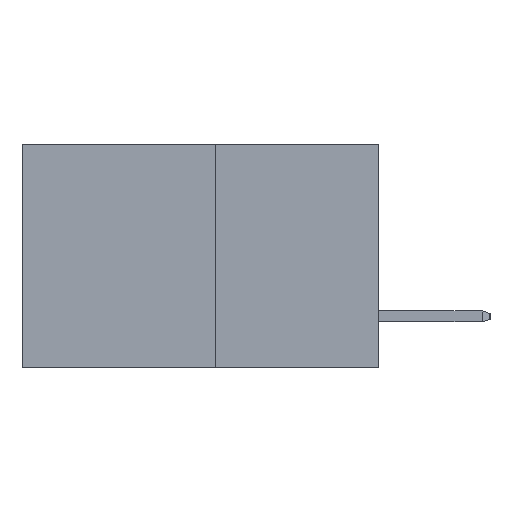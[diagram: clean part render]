
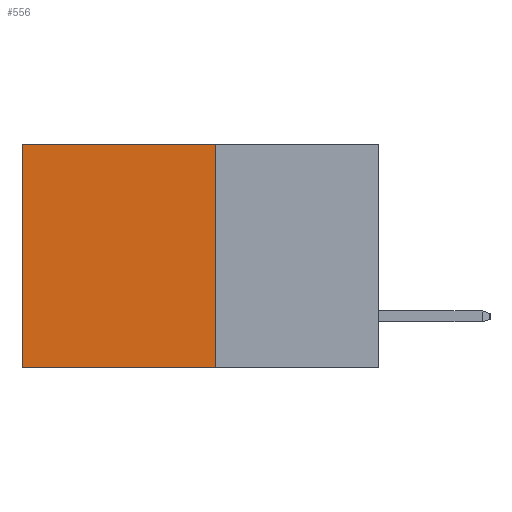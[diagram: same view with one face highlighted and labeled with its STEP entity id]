
A CAD part, left-side view. The second image highlights one B-rep face of the part: STEP entity #556.
In plain terms, the highlighted planar face has unit normal (-1, 0, 0).
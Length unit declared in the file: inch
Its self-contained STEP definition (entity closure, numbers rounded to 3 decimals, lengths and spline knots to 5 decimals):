
#320 = VERTEX_POINT ( 'NONE', #10643 ) ;
#556 = ADVANCED_FACE ( 'NONE', ( #1606 ), #7181, .F. ) ;
#638 = DIRECTION ( 'NONE',  ( 0., 0., -1. ) ) ;
#1606 = FACE_OUTER_BOUND ( 'NONE', #9519, .T. ) ;
#1773 = EDGE_CURVE ( 'NONE', #8562, #7394, #2162, .T. ) ;
#1895 = DIRECTION ( 'NONE',  ( 1., 0., 0. ) ) ;
#2162 = LINE ( 'NONE', #6145, #2445 ) ;
#2347 = LINE ( 'NONE', #3818, #9650 ) ;
#2445 = VECTOR ( 'NONE', #6106, 39.37008 ) ;
#2896 = ORIENTED_EDGE ( 'NONE', *, *, #3645, .T. ) ;
#3191 = ORIENTED_EDGE ( 'NONE', *, *, #10747, .T. ) ;
#3645 = EDGE_CURVE ( 'NONE', #320, #7394, #4684, .T. ) ;
#3818 = CARTESIAN_POINT ( 'NONE',  ( 0.277, 0.27, 0. ) ) ;
#4272 = CARTESIAN_POINT ( 'NONE',  ( 0.277, 0.27, -0.37 ) ) ;
#4500 = VERTEX_POINT ( 'NONE', #7569 ) ;
#4599 = LINE ( 'NONE', #6150, #9473 ) ;
#4684 = LINE ( 'NONE', #7059, #11668 ) ;
#5683 = CARTESIAN_POINT ( 'NONE',  ( 0.277, 0.59, -0.37 ) ) ;
#6106 = DIRECTION ( 'NONE',  ( 0., 1., 0. ) ) ;
#6145 = CARTESIAN_POINT ( 'NONE',  ( 0.277, 0.27, -0.37 ) ) ;
#6150 = CARTESIAN_POINT ( 'NONE',  ( 0.277, 0.27, -0.37 ) ) ;
#7001 = EDGE_CURVE ( 'NONE', #4500, #8562, #4599, .T. ) ;
#7059 = CARTESIAN_POINT ( 'NONE',  ( 0.277, 0.59, -0.37 ) ) ;
#7181 = PLANE ( 'NONE',  #11571 ) ;
#7394 = VERTEX_POINT ( 'NONE', #5683 ) ;
#7569 = CARTESIAN_POINT ( 'NONE',  ( 0.277, 0.27, 0. ) ) ;
#7791 = ORIENTED_EDGE ( 'NONE', *, *, #1773, .F. ) ;
#8096 = DIRECTION ( 'NONE',  ( 0., 0., -1. ) ) ;
#8562 = VERTEX_POINT ( 'NONE', #10236 ) ;
#9473 = VECTOR ( 'NONE', #638, 39.37008 ) ;
#9519 = EDGE_LOOP ( 'NONE', ( #2896, #7791, #10185, #3191 ) ) ;
#9650 = VECTOR ( 'NONE', #11109, 39.37008 ) ;
#9825 = DIRECTION ( 'NONE',  ( 0., 0., -1. ) ) ;
#10185 = ORIENTED_EDGE ( 'NONE', *, *, #7001, .F. ) ;
#10236 = CARTESIAN_POINT ( 'NONE',  ( 0.277, 0.27, -0.37 ) ) ;
#10643 = CARTESIAN_POINT ( 'NONE',  ( 0.277, 0.59, 0. ) ) ;
#10747 = EDGE_CURVE ( 'NONE', #4500, #320, #2347, .T. ) ;
#11109 = DIRECTION ( 'NONE',  ( 0., 1., 0. ) ) ;
#11571 = AXIS2_PLACEMENT_3D ( 'NONE', #4272, #1895, #8096 ) ;
#11668 = VECTOR ( 'NONE', #9825, 39.37008 ) ;
